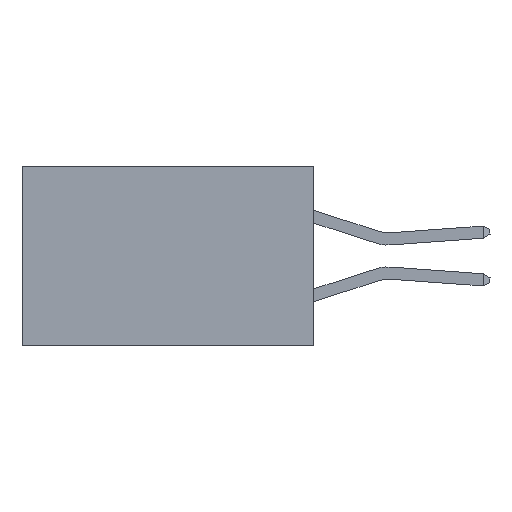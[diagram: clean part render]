
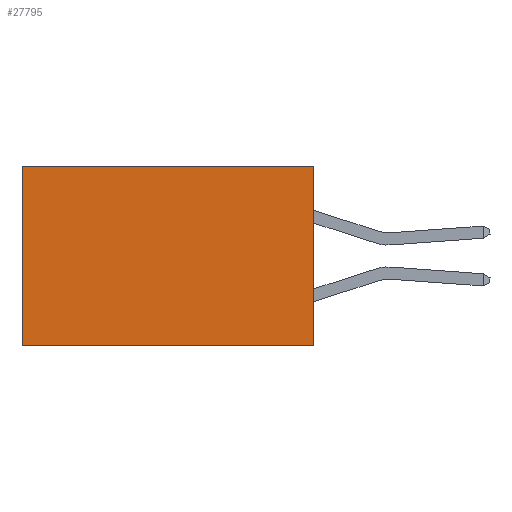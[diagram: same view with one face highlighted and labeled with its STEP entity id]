
A CAD part, left-side view. The second image highlights one B-rep face of the part: STEP entity #27795.
In plain terms, the highlighted planar face has unit normal (-1, 0, 0).
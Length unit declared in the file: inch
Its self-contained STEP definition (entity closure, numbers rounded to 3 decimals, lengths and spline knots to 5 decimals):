
#231 = EDGE_CURVE ( 'NONE', #16969, #673, #27686, .T. ) ;
#673 = VERTEX_POINT ( 'NONE', #13854 ) ;
#837 = CARTESIAN_POINT ( 'NONE',  ( 0.2875, 0., 0. ) ) ;
#1480 = CARTESIAN_POINT ( 'NONE',  ( 0.2875, 0., -0.37 ) ) ;
#4072 = CARTESIAN_POINT ( 'NONE',  ( 0.2875, 0., 0. ) ) ;
#4343 = CARTESIAN_POINT ( 'NONE',  ( 0.2875, 0.6, 0. ) ) ;
#4466 = AXIS2_PLACEMENT_3D ( 'NONE', #5527, #23651, #12016 ) ;
#5527 = CARTESIAN_POINT ( 'NONE',  ( 0.2875, 0., 0. ) ) ;
#5779 = DIRECTION ( 'NONE',  ( 0., 0., -1. ) ) ;
#6075 = CARTESIAN_POINT ( 'NONE',  ( 0.2875, 0., 0. ) ) ;
#7757 = LINE ( 'NONE', #32095, #13197 ) ;
#11022 = CARTESIAN_POINT ( 'NONE',  ( 0.2875, 0., -0.37 ) ) ;
#12016 = DIRECTION ( 'NONE',  ( 0., 0., -1. ) ) ;
#13197 = VECTOR ( 'NONE', #5779, 39.37008 ) ;
#13854 = CARTESIAN_POINT ( 'NONE',  ( 0.2875, 0.6, -0.37 ) ) ;
#16086 = ORIENTED_EDGE ( 'NONE', *, *, #31758, .T. ) ;
#16969 = VERTEX_POINT ( 'NONE', #11022 ) ;
#17130 = VERTEX_POINT ( 'NONE', #4343 ) ;
#19444 = PLANE ( 'NONE',  #4466 ) ;
#19741 = ORIENTED_EDGE ( 'NONE', *, *, #32510, .F. ) ;
#19744 = VERTEX_POINT ( 'NONE', #837 ) ;
#21974 = ORIENTED_EDGE ( 'NONE', *, *, #231, .F. ) ;
#23651 = DIRECTION ( 'NONE',  ( 1., 0., 0. ) ) ;
#24971 = VECTOR ( 'NONE', #36253, 39.37008 ) ;
#26744 = DIRECTION ( 'NONE',  ( 0., 1., 0. ) ) ;
#27512 = DIRECTION ( 'NONE',  ( 0., 0., -1. ) ) ;
#27674 = EDGE_LOOP ( 'NONE', ( #34324, #21974, #19741, #16086 ) ) ;
#27686 = LINE ( 'NONE', #1480, #24971 ) ;
#27795 = ADVANCED_FACE ( 'NONE', ( #30871 ), #19444, .F. ) ;
#28903 = EDGE_CURVE ( 'NONE', #17130, #673, #7757, .T. ) ;
#30871 = FACE_OUTER_BOUND ( 'NONE', #27674, .T. ) ;
#30944 = LINE ( 'NONE', #4072, #32232 ) ;
#31000 = LINE ( 'NONE', #6075, #33252 ) ;
#31758 = EDGE_CURVE ( 'NONE', #19744, #17130, #31000, .T. ) ;
#32095 = CARTESIAN_POINT ( 'NONE',  ( 0.2875, 0.6, 0. ) ) ;
#32232 = VECTOR ( 'NONE', #27512, 39.37008 ) ;
#32510 = EDGE_CURVE ( 'NONE', #19744, #16969, #30944, .T. ) ;
#33252 = VECTOR ( 'NONE', #26744, 39.37008 ) ;
#34324 = ORIENTED_EDGE ( 'NONE', *, *, #28903, .T. ) ;
#36253 = DIRECTION ( 'NONE',  ( 0., 1., 0. ) ) ;
